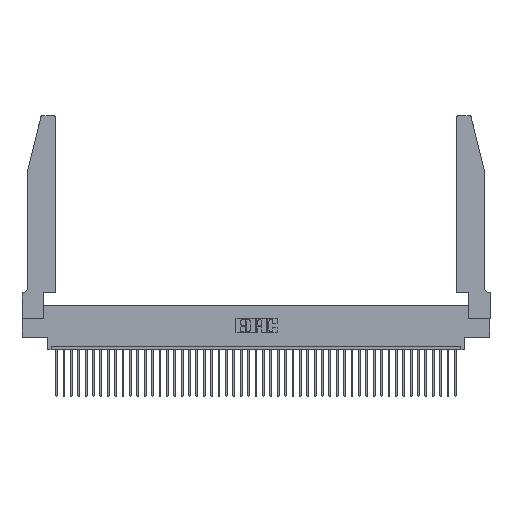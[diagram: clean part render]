
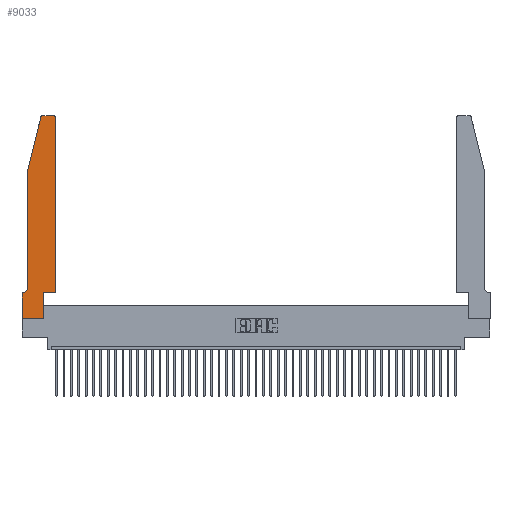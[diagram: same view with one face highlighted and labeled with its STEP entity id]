
A CAD part, top view. The second image highlights one B-rep face of the part: STEP entity #9033.
In plain terms, the highlighted planar face has unit normal (0, 0, 1).
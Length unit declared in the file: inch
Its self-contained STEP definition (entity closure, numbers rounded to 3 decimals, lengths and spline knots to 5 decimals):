
#802 = VECTOR ( 'NONE', #9183, 39.37008 ) ;
#1163 = EDGE_CURVE ( 'NONE', #40392, #40047, #27909, .T. ) ;
#1647 = CARTESIAN_POINT ( 'NONE',  ( 0.2865, 0., 0.37 ) ) ;
#1945 = ORIENTED_EDGE ( 'NONE', *, *, #4396, .T. ) ;
#1959 = CARTESIAN_POINT ( 'NONE',  ( 0.25487, 2.72718, 0.37 ) ) ;
#2368 = CARTESIAN_POINT ( 'NONE',  ( 0.2605, 2.75, 0.37 ) ) ;
#2582 = CARTESIAN_POINT ( 'NONE',  ( 0., 0.35, 0.37 ) ) ;
#3048 = CARTESIAN_POINT ( 'NONE',  ( 0.4205, 2.72, 0.37 ) ) ;
#3065 = EDGE_CURVE ( 'NONE', #4226, #9970, #7758, .T. ) ;
#3237 = DIRECTION ( 'NONE',  ( -0.239, -0.971, 0. ) ) ;
#3261 = DIRECTION ( 'NONE',  ( 0., 0., -1. ) ) ;
#3848 = DIRECTION ( 'NONE',  ( 0., 0., 1. ) ) ;
#4226 = VERTEX_POINT ( 'NONE', #1647 ) ;
#4396 = EDGE_CURVE ( 'NONE', #9970, #5748, #10404, .T. ) ;
#4714 = DIRECTION ( 'NONE',  ( -1., 0., 0. ) ) ;
#5748 = VERTEX_POINT ( 'NONE', #33720 ) ;
#6018 = PLANE ( 'NONE',  #40327 ) ;
#6381 = EDGE_CURVE ( 'NONE', #34461, #14121, #41831, .T. ) ;
#6864 = ORIENTED_EDGE ( 'NONE', *, *, #6381, .T. ) ;
#6883 = CARTESIAN_POINT ( 'NONE',  ( 0.0755, 2., 0.37 ) ) ;
#6952 = VECTOR ( 'NONE', #13634, 39.37008 ) ;
#7284 = DIRECTION ( 'NONE',  ( 1., 0., 0. ) ) ;
#7758 = LINE ( 'NONE', #16589, #37911 ) ;
#8414 = CARTESIAN_POINT ( 'NONE',  ( 0.2865, 0.35, 0.37 ) ) ;
#8977 = ORIENTED_EDGE ( 'NONE', *, *, #40888, .T. ) ;
#9033 = ADVANCED_FACE ( 'NONE', ( #11962 ), #6018, .T. ) ;
#9183 = DIRECTION ( 'NONE',  ( -1., 0., 0. ) ) ;
#9375 = ORIENTED_EDGE ( 'NONE', *, *, #1163, .T. ) ;
#9970 = VERTEX_POINT ( 'NONE', #8414 ) ;
#10082 = VERTEX_POINT ( 'NONE', #15197 ) ;
#10217 = CARTESIAN_POINT ( 'NONE',  ( 0.284, 2.75, 0.37 ) ) ;
#10404 = LINE ( 'NONE', #44356, #24444 ) ;
#10415 = ORIENTED_EDGE ( 'NONE', *, *, #33551, .T. ) ;
#10455 = CIRCLE ( 'NONE', #33270, 0.03 ) ;
#11025 = DIRECTION ( 'NONE',  ( 1., 0., 0. ) ) ;
#11089 = CARTESIAN_POINT ( 'NONE',  ( 0.284, 2.72, 0.37 ) ) ;
#11962 = FACE_OUTER_BOUND ( 'NONE', #20890, .T. ) ;
#12599 = EDGE_CURVE ( 'NONE', #10082, #4226, #28079, .T. ) ;
#13386 = VECTOR ( 'NONE', #4714, 39.37008 ) ;
#13421 = ORIENTED_EDGE ( 'NONE', *, *, #30016, .T. ) ;
#13538 = CARTESIAN_POINT ( 'NONE',  ( 0., 0.35, 0.37 ) ) ;
#13634 = DIRECTION ( 'NONE',  ( 0., 1., 0. ) ) ;
#13666 = AXIS2_PLACEMENT_3D ( 'NONE', #3048, #14363, #21286 ) ;
#13878 = ORIENTED_EDGE ( 'NONE', *, *, #3065, .T. ) ;
#13943 = DIRECTION ( 'NONE',  ( 1., 0., 0. ) ) ;
#14121 = VERTEX_POINT ( 'NONE', #16381 ) ;
#14363 = DIRECTION ( 'NONE',  ( 0., 0., 1. ) ) ;
#14583 = CARTESIAN_POINT ( 'NONE',  ( 0.4505, 2.72, 0.37 ) ) ;
#15197 = CARTESIAN_POINT ( 'NONE',  ( 0., 0., 0.37 ) ) ;
#16103 = LINE ( 'NONE', #37248, #6952 ) ;
#16381 = CARTESIAN_POINT ( 'NONE',  ( 0.0755, 0.42, 0.37 ) ) ;
#16447 = VECTOR ( 'NONE', #3237, 39.37008 ) ;
#16589 = CARTESIAN_POINT ( 'NONE',  ( 0.2865, 0.35, 0.37 ) ) ;
#16635 = EDGE_CURVE ( 'NONE', #39436, #10082, #39519, .T. ) ;
#18138 = VERTEX_POINT ( 'NONE', #1959 ) ;
#18291 = LINE ( 'NONE', #25380, #13386 ) ;
#20890 = EDGE_LOOP ( 'NONE', ( #10415, #8977, #25457, #6864, #41721, #23456, #35584, #33133, #13878, #1945, #13421, #9375 ) ) ;
#21286 = DIRECTION ( 'NONE',  ( 1., 0., 0. ) ) ;
#22692 = VERTEX_POINT ( 'NONE', #10217 ) ;
#22952 = DIRECTION ( 'NONE',  ( 0., 1., 0. ) ) ;
#23247 = VECTOR ( 'NONE', #29401, 39.37008 ) ;
#23261 = CARTESIAN_POINT ( 'NONE',  ( 0.0755, 2., 0.37 ) ) ;
#23456 = ORIENTED_EDGE ( 'NONE', *, *, #43835, .T. ) ;
#23497 = LINE ( 'NONE', #6883, #16447 ) ;
#23670 = CARTESIAN_POINT ( 'NONE',  ( 0.0755, 2., 0.37 ) ) ;
#24444 = VECTOR ( 'NONE', #11025, 39.37008 ) ;
#25380 = CARTESIAN_POINT ( 'NONE',  ( 0.0755, 0.35, 0.37 ) ) ;
#25457 = ORIENTED_EDGE ( 'NONE', *, *, #26056, .T. ) ;
#26056 = EDGE_CURVE ( 'NONE', #18138, #34461, #23497, .T. ) ;
#26572 = DIRECTION ( 'NONE',  ( 0., -1., 0. ) ) ;
#27277 = DIRECTION ( 'NONE',  ( -1., 0., 0. ) ) ;
#27909 = CIRCLE ( 'NONE', #13666, 0.03 ) ;
#28079 = LINE ( 'NONE', #35096, #23247 ) ;
#29401 = DIRECTION ( 'NONE',  ( 1., 0., 0. ) ) ;
#29457 = CARTESIAN_POINT ( 'NONE',  ( 0., 0., 0.37 ) ) ;
#30016 = EDGE_CURVE ( 'NONE', #5748, #40392, #16103, .T. ) ;
#32677 = VECTOR ( 'NONE', #26572, 39.37008 ) ;
#33133 = ORIENTED_EDGE ( 'NONE', *, *, #12599, .T. ) ;
#33270 = AXIS2_PLACEMENT_3D ( 'NONE', #11089, #3848, #13943 ) ;
#33489 = CIRCLE ( 'NONE', #38384, 0.07 ) ;
#33551 = EDGE_CURVE ( 'NONE', #40047, #22692, #36349, .T. ) ;
#33714 = CARTESIAN_POINT ( 'NONE',  ( 0.4205, 2.75, 0.37 ) ) ;
#33720 = CARTESIAN_POINT ( 'NONE',  ( 0.4505, 0.35, 0.37 ) ) ;
#34461 = VERTEX_POINT ( 'NONE', #23670 ) ;
#34714 = DIRECTION ( 'NONE',  ( 0., 0., 1. ) ) ;
#35096 = CARTESIAN_POINT ( 'NONE',  ( 0., 0., 0.37 ) ) ;
#35275 = EDGE_CURVE ( 'NONE', #14121, #41914, #33489, .T. ) ;
#35584 = ORIENTED_EDGE ( 'NONE', *, *, #16635, .T. ) ;
#36345 = DIRECTION ( 'NONE',  ( 0., -1., 0. ) ) ;
#36349 = LINE ( 'NONE', #2368, #802 ) ;
#37248 = CARTESIAN_POINT ( 'NONE',  ( 0.4505, 0.35, 0.37 ) ) ;
#37911 = VECTOR ( 'NONE', #22952, 39.37008 ) ;
#37914 = VECTOR ( 'NONE', #36345, 39.37008 ) ;
#38384 = AXIS2_PLACEMENT_3D ( 'NONE', #44297, #3261, #27277 ) ;
#39436 = VERTEX_POINT ( 'NONE', #2582 ) ;
#39519 = LINE ( 'NONE', #29457, #37914 ) ;
#40047 = VERTEX_POINT ( 'NONE', #33714 ) ;
#40327 = AXIS2_PLACEMENT_3D ( 'NONE', #13538, #34714, #7284 ) ;
#40392 = VERTEX_POINT ( 'NONE', #14583 ) ;
#40888 = EDGE_CURVE ( 'NONE', #22692, #18138, #10455, .T. ) ;
#41721 = ORIENTED_EDGE ( 'NONE', *, *, #35275, .T. ) ;
#41831 = LINE ( 'NONE', #23261, #32677 ) ;
#41914 = VERTEX_POINT ( 'NONE', #44156 ) ;
#43835 = EDGE_CURVE ( 'NONE', #41914, #39436, #18291, .T. ) ;
#44156 = CARTESIAN_POINT ( 'NONE',  ( 0.0055, 0.35, 0.37 ) ) ;
#44297 = CARTESIAN_POINT ( 'NONE',  ( 0.0055, 0.42, 0.37 ) ) ;
#44356 = CARTESIAN_POINT ( 'NONE',  ( 0.4505, 0.35, 0.37 ) ) ;
